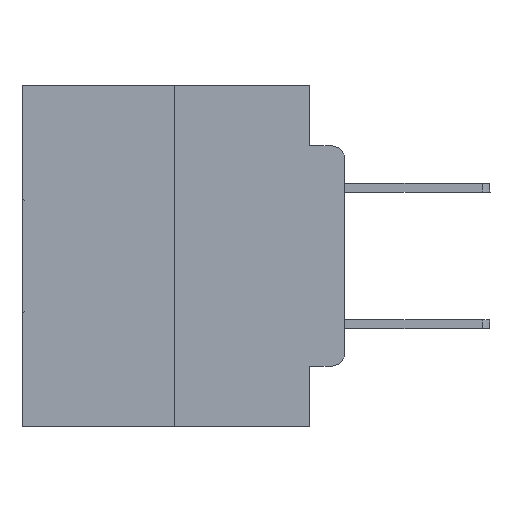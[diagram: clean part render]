
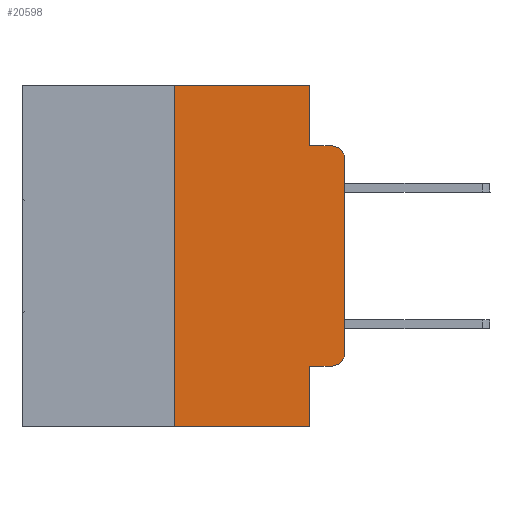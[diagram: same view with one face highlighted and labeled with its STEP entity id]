
A CAD part, left-side view. The second image highlights one B-rep face of the part: STEP entity #20598.
In plain terms, the highlighted planar face has unit normal (-1, 0, 0).
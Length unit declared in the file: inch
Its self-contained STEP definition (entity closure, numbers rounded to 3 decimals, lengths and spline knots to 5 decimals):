
#420 = VECTOR ( 'NONE', #17709, 39.37008 ) ;
#647 = CARTESIAN_POINT ( 'NONE',  ( 0., 0.473, 0. ) ) ;
#886 = ORIENTED_EDGE ( 'NONE', *, *, #2685, .T. ) ;
#896 = CARTESIAN_POINT ( 'NONE',  ( 0., 0.02, -0.0885 ) ) ;
#1044 = AXIS2_PLACEMENT_3D ( 'NONE', #19381, #14455, #23397 ) ;
#1224 = CARTESIAN_POINT ( 'NONE',  ( 0., 0.051, -0.4115 ) ) ;
#2078 = LINE ( 'NONE', #21180, #22766 ) ;
#2375 = DIRECTION ( 'NONE',  ( 0., 0., 1. ) ) ;
#2685 = EDGE_CURVE ( 'NONE', #13693, #18702, #8936, .T. ) ;
#3121 = LINE ( 'NONE', #19758, #23803 ) ;
#3122 = DIRECTION ( 'NONE',  ( 0., -1., 0. ) ) ;
#3947 = CARTESIAN_POINT ( 'NONE',  ( 0., 0.473, 0. ) ) ;
#4485 = EDGE_CURVE ( 'NONE', #20948, #18702, #15338, .T. ) ;
#5032 = DIRECTION ( 'NONE',  ( 0., 0., -1. ) ) ;
#6190 = ORIENTED_EDGE ( 'NONE', *, *, #19378, .F. ) ;
#6614 = CARTESIAN_POINT ( 'NONE',  ( 0., 0., -0.3915 ) ) ;
#6807 = CARTESIAN_POINT ( 'NONE',  ( 0., 0.051, 0. ) ) ;
#7350 = VECTOR ( 'NONE', #3122, 39.37008 ) ;
#8163 = LINE ( 'NONE', #15862, #420 ) ;
#8235 = CARTESIAN_POINT ( 'NONE',  ( 0., 0.051, -0.0885 ) ) ;
#8936 = CIRCLE ( 'NONE', #1044, 0.02 ) ;
#9136 = VERTEX_POINT ( 'NONE', #12435 ) ;
#9431 = CARTESIAN_POINT ( 'NONE',  ( 0., 0.051, -0.4115 ) ) ;
#10221 = DIRECTION ( 'NONE',  ( 0., 0., -1. ) ) ;
#10333 = CARTESIAN_POINT ( 'NONE',  ( 0., 0.051, -0.5 ) ) ;
#10856 = ORIENTED_EDGE ( 'NONE', *, *, #14036, .T. ) ;
#11000 = VERTEX_POINT ( 'NONE', #29688 ) ;
#11073 = ORIENTED_EDGE ( 'NONE', *, *, #18275, .T. ) ;
#11076 = DIRECTION ( 'NONE',  ( 0., 0., 1. ) ) ;
#11793 = EDGE_CURVE ( 'NONE', #26320, #21346, #3121, .T. ) ;
#12435 = CARTESIAN_POINT ( 'NONE',  ( 0., 0.02, -0.4115 ) ) ;
#13604 = VECTOR ( 'NONE', #14061, 39.37008 ) ;
#13693 = VERTEX_POINT ( 'NONE', #29886 ) ;
#14036 = EDGE_CURVE ( 'NONE', #9136, #18638, #22951, .T. ) ;
#14061 = DIRECTION ( 'NONE',  ( 0., 0., -1. ) ) ;
#14455 = DIRECTION ( 'NONE',  ( -1., 0., 0. ) ) ;
#14837 = ORIENTED_EDGE ( 'NONE', *, *, #23383, .T. ) ;
#14848 = ORIENTED_EDGE ( 'NONE', *, *, #11793, .F. ) ;
#15128 = AXIS2_PLACEMENT_3D ( 'NONE', #3947, #15818, #29210 ) ;
#15338 = LINE ( 'NONE', #24747, #26964 ) ;
#15360 = PLANE ( 'NONE',  #15128 ) ;
#15401 = LINE ( 'NONE', #1224, #21890 ) ;
#15659 = FACE_OUTER_BOUND ( 'NONE', #20667, .T. ) ;
#15818 = DIRECTION ( 'NONE',  ( 1., 0., 0. ) ) ;
#15845 = CARTESIAN_POINT ( 'NONE',  ( 0., 0.25, 0. ) ) ;
#15862 = CARTESIAN_POINT ( 'NONE',  ( 0., 0.473, -0.5 ) ) ;
#16497 = ORIENTED_EDGE ( 'NONE', *, *, #22807, .F. ) ;
#17139 = LINE ( 'NONE', #647, #7350 ) ;
#17709 = DIRECTION ( 'NONE',  ( 0., -1., 0. ) ) ;
#18275 = EDGE_CURVE ( 'NONE', #26320, #9136, #15401, .T. ) ;
#18638 = VERTEX_POINT ( 'NONE', #6614 ) ;
#18702 = VERTEX_POINT ( 'NONE', #896 ) ;
#18834 = EDGE_CURVE ( 'NONE', #24545, #29445, #19850, .T. ) ;
#19378 = EDGE_CURVE ( 'NONE', #11000, #20948, #28377, .T. ) ;
#19381 = CARTESIAN_POINT ( 'NONE',  ( 0., 0.02, -0.1085 ) ) ;
#19463 = VECTOR ( 'NONE', #11076, 39.37008 ) ;
#19511 = CARTESIAN_POINT ( 'NONE',  ( 0., 0.02, -0.3915 ) ) ;
#19758 = CARTESIAN_POINT ( 'NONE',  ( 0., 0.051, 0. ) ) ;
#19850 = LINE ( 'NONE', #15845, #19463 ) ;
#19866 = DIRECTION ( 'NONE',  ( 0., -1., 0. ) ) ;
#20598 = ADVANCED_FACE ( 'NONE', ( #15659 ), #15360, .F. ) ;
#20667 = EDGE_LOOP ( 'NONE', ( #21945, #886, #27618, #6190, #16497, #27929, #14837, #14848, #11073, #10856 ) ) ;
#20948 = VERTEX_POINT ( 'NONE', #8235 ) ;
#21180 = CARTESIAN_POINT ( 'NONE',  ( 0., 0., 0. ) ) ;
#21346 = VERTEX_POINT ( 'NONE', #10333 ) ;
#21690 = DIRECTION ( 'NONE',  ( -1., 0., 0. ) ) ;
#21890 = VECTOR ( 'NONE', #19866, 39.37008 ) ;
#21945 = ORIENTED_EDGE ( 'NONE', *, *, #26762, .T. ) ;
#22766 = VECTOR ( 'NONE', #2375, 39.37008 ) ;
#22807 = EDGE_CURVE ( 'NONE', #29445, #11000, #17139, .T. ) ;
#22951 = CIRCLE ( 'NONE', #23908, 0.02 ) ;
#23383 = EDGE_CURVE ( 'NONE', #24545, #21346, #8163, .T. ) ;
#23397 = DIRECTION ( 'NONE',  ( 0., 0., -1. ) ) ;
#23803 = VECTOR ( 'NONE', #10221, 39.37008 ) ;
#23908 = AXIS2_PLACEMENT_3D ( 'NONE', #19511, #21690, #5032 ) ;
#24058 = CARTESIAN_POINT ( 'NONE',  ( 0., 0.25, -0.5 ) ) ;
#24545 = VERTEX_POINT ( 'NONE', #24058 ) ;
#24747 = CARTESIAN_POINT ( 'NONE',  ( 0., 0.051, -0.0885 ) ) ;
#26320 = VERTEX_POINT ( 'NONE', #9431 ) ;
#26762 = EDGE_CURVE ( 'NONE', #18638, #13693, #2078, .T. ) ;
#26964 = VECTOR ( 'NONE', #28890, 39.37008 ) ;
#27618 = ORIENTED_EDGE ( 'NONE', *, *, #4485, .F. ) ;
#27929 = ORIENTED_EDGE ( 'NONE', *, *, #18834, .F. ) ;
#28106 = CARTESIAN_POINT ( 'NONE',  ( 0., 0.25, 0. ) ) ;
#28377 = LINE ( 'NONE', #6807, #13604 ) ;
#28890 = DIRECTION ( 'NONE',  ( 0., -1., 0. ) ) ;
#29210 = DIRECTION ( 'NONE',  ( 0., 0., -1. ) ) ;
#29445 = VERTEX_POINT ( 'NONE', #28106 ) ;
#29688 = CARTESIAN_POINT ( 'NONE',  ( 0., 0.051, 0. ) ) ;
#29886 = CARTESIAN_POINT ( 'NONE',  ( 0., 0., -0.1085 ) ) ;
